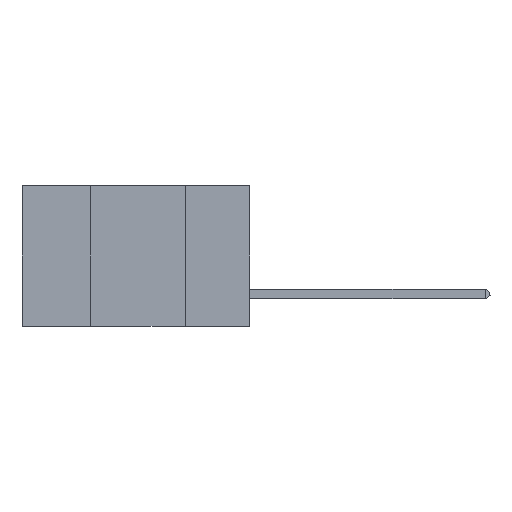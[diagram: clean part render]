
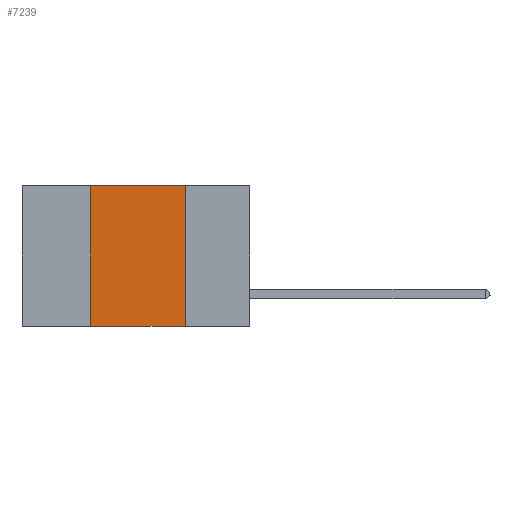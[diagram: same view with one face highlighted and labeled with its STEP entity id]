
A CAD part, left-side view. The second image highlights one B-rep face of the part: STEP entity #7239.
In plain terms, the highlighted planar face has unit normal (-1, 0, 0).
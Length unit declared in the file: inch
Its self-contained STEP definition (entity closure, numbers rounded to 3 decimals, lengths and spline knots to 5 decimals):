
#344 = CARTESIAN_POINT ( 'NONE',  ( 0., 0.17, 0. ) ) ;
#436 = VERTEX_POINT ( 'NONE', #10439 ) ;
#557 = ORIENTED_EDGE ( 'NONE', *, *, #9056, .T. ) ;
#889 = EDGE_CURVE ( 'NONE', #436, #5212, #3447, .T. ) ;
#1269 = DIRECTION ( 'NONE',  ( 0., 0., -1. ) ) ;
#2167 = CARTESIAN_POINT ( 'NONE',  ( 0., 0.17, -0.37 ) ) ;
#2640 = DIRECTION ( 'NONE',  ( 0., 0., 1. ) ) ;
#2681 = VERTEX_POINT ( 'NONE', #2167 ) ;
#2770 = AXIS2_PLACEMENT_3D ( 'NONE', #3968, #5901, #6877 ) ;
#2895 = CARTESIAN_POINT ( 'NONE',  ( 0., 0.42, 0. ) ) ;
#2954 = CARTESIAN_POINT ( 'NONE',  ( 0., 0.6, -0.37 ) ) ;
#3447 = LINE ( 'NONE', #6479, #5106 ) ;
#3630 = ORIENTED_EDGE ( 'NONE', *, *, #889, .F. ) ;
#3882 = VERTEX_POINT ( 'NONE', #344 ) ;
#3883 = PLANE ( 'NONE',  #2770 ) ;
#3968 = CARTESIAN_POINT ( 'NONE',  ( 0., 0.6, 0. ) ) ;
#5106 = VECTOR ( 'NONE', #2640, 39.37008 ) ;
#5212 = VERTEX_POINT ( 'NONE', #2895 ) ;
#5884 = DIRECTION ( 'NONE',  ( 0., -1., 0. ) ) ;
#5901 = DIRECTION ( 'NONE',  ( 1., 0., 0. ) ) ;
#6479 = CARTESIAN_POINT ( 'NONE',  ( 0., 0.42, 0. ) ) ;
#6843 = ORIENTED_EDGE ( 'NONE', *, *, #8706, .F. ) ;
#6877 = DIRECTION ( 'NONE',  ( 0., 0., -1. ) ) ;
#7239 = ADVANCED_FACE ( 'NONE', ( #9212 ), #3883, .F. ) ;
#7319 = VECTOR ( 'NONE', #11739, 39.37008 ) ;
#7690 = EDGE_CURVE ( 'NONE', #5212, #3882, #9954, .T. ) ;
#8706 = EDGE_CURVE ( 'NONE', #3882, #2681, #9462, .T. ) ;
#9056 = EDGE_CURVE ( 'NONE', #436, #2681, #10831, .T. ) ;
#9212 = FACE_OUTER_BOUND ( 'NONE', #11927, .T. ) ;
#9320 = VECTOR ( 'NONE', #1269, 39.37008 ) ;
#9342 = VECTOR ( 'NONE', #5884, 39.37008 ) ;
#9462 = LINE ( 'NONE', #10949, #9320 ) ;
#9842 = CARTESIAN_POINT ( 'NONE',  ( 0., 0.6, 0. ) ) ;
#9954 = LINE ( 'NONE', #9842, #9342 ) ;
#10439 = CARTESIAN_POINT ( 'NONE',  ( 0., 0.42, -0.37 ) ) ;
#10502 = ORIENTED_EDGE ( 'NONE', *, *, #7690, .F. ) ;
#10831 = LINE ( 'NONE', #2954, #7319 ) ;
#10949 = CARTESIAN_POINT ( 'NONE',  ( 0., 0.17, 0. ) ) ;
#11739 = DIRECTION ( 'NONE',  ( 0., -1., 0. ) ) ;
#11927 = EDGE_LOOP ( 'NONE', ( #6843, #10502, #3630, #557 ) ) ;
